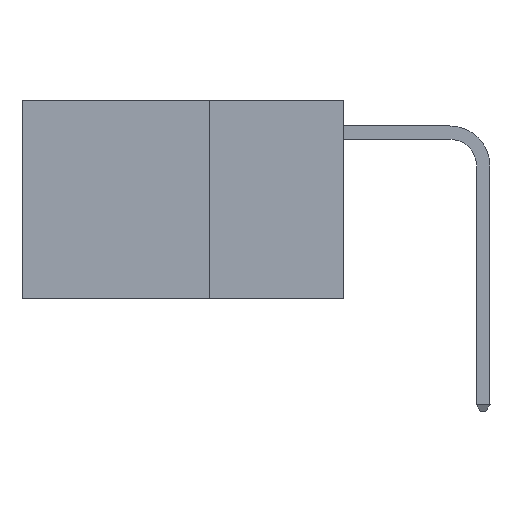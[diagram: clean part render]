
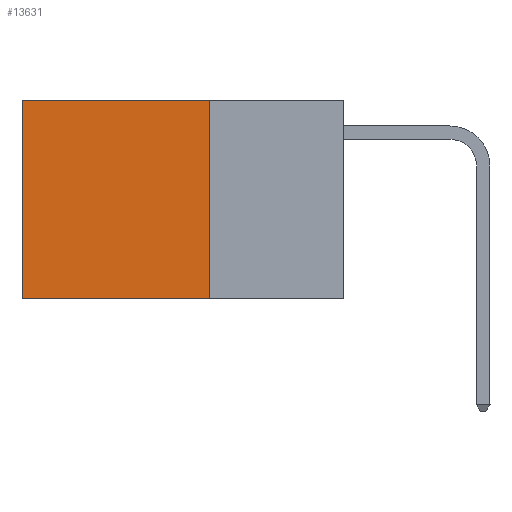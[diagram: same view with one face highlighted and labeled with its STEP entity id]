
A CAD part, left-side view. The second image highlights one B-rep face of the part: STEP entity #13631.
In plain terms, the highlighted planar face has unit normal (-1, 0, 0).
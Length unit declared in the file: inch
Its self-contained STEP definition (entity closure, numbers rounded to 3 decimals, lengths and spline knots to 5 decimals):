
#1670 = PLANE ( 'NONE',  #26466 ) ;
#3205 = ORIENTED_EDGE ( 'NONE', *, *, #10557, .F. ) ;
#4611 = ORIENTED_EDGE ( 'NONE', *, *, #15492, .T. ) ;
#4881 = CARTESIAN_POINT ( 'NONE',  ( 0.2625, 0.25, 0. ) ) ;
#6248 = LINE ( 'NONE', #8829, #17230 ) ;
#6267 = VECTOR ( 'NONE', #11878, 39.37008 ) ;
#7834 = ORIENTED_EDGE ( 'NONE', *, *, #17530, .T. ) ;
#8317 = VERTEX_POINT ( 'NONE', #19051 ) ;
#8829 = CARTESIAN_POINT ( 'NONE',  ( 0.2625, 0.25, 0. ) ) ;
#8977 = CARTESIAN_POINT ( 'NONE',  ( 0.2625, 0.25, 0. ) ) ;
#9462 = DIRECTION ( 'NONE',  ( 0., 0., -1. ) ) ;
#10020 = CARTESIAN_POINT ( 'NONE',  ( 0.2625, 0.25, -0.37 ) ) ;
#10557 = EDGE_CURVE ( 'NONE', #20150, #13051, #16995, .T. ) ;
#10992 = DIRECTION ( 'NONE',  ( 0., 0., -1. ) ) ;
#11878 = DIRECTION ( 'NONE',  ( 0., 1., 0. ) ) ;
#12179 = CARTESIAN_POINT ( 'NONE',  ( 0.2625, 0.25, -0.37 ) ) ;
#13051 = VERTEX_POINT ( 'NONE', #10020 ) ;
#13631 = ADVANCED_FACE ( 'NONE', ( #17781 ), #1670, .F. ) ;
#14017 = LINE ( 'NONE', #12179, #6267 ) ;
#15428 = VERTEX_POINT ( 'NONE', #27366 ) ;
#15492 = EDGE_CURVE ( 'NONE', #20150, #8317, #6248, .T. ) ;
#15795 = DIRECTION ( 'NONE',  ( 0., 0., -1. ) ) ;
#16995 = LINE ( 'NONE', #4881, #19042 ) ;
#17230 = VECTOR ( 'NONE', #27067, 39.37008 ) ;
#17530 = EDGE_CURVE ( 'NONE', #8317, #15428, #27057, .T. ) ;
#17781 = FACE_OUTER_BOUND ( 'NONE', #19283, .T. ) ;
#19042 = VECTOR ( 'NONE', #9462, 39.37008 ) ;
#19051 = CARTESIAN_POINT ( 'NONE',  ( 0.2625, 0.6, 0. ) ) ;
#19283 = EDGE_LOOP ( 'NONE', ( #7834, #24504, #3205, #4611 ) ) ;
#20150 = VERTEX_POINT ( 'NONE', #8977 ) ;
#20374 = CARTESIAN_POINT ( 'NONE',  ( 0.2625, 0.25, 0. ) ) ;
#20713 = VECTOR ( 'NONE', #10992, 39.37008 ) ;
#23045 = EDGE_CURVE ( 'NONE', #13051, #15428, #14017, .T. ) ;
#24504 = ORIENTED_EDGE ( 'NONE', *, *, #23045, .F. ) ;
#24921 = CARTESIAN_POINT ( 'NONE',  ( 0.2625, 0.6, 0. ) ) ;
#26466 = AXIS2_PLACEMENT_3D ( 'NONE', #20374, #27096, #15795 ) ;
#27057 = LINE ( 'NONE', #24921, #20713 ) ;
#27067 = DIRECTION ( 'NONE',  ( 0., 1., 0. ) ) ;
#27096 = DIRECTION ( 'NONE',  ( 1., 0., 0. ) ) ;
#27366 = CARTESIAN_POINT ( 'NONE',  ( 0.2625, 0.6, -0.37 ) ) ;
